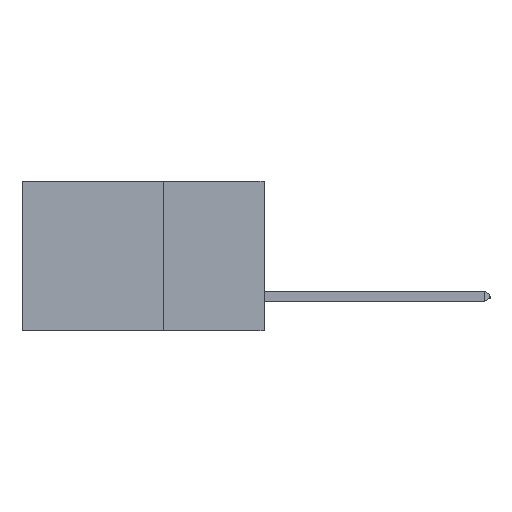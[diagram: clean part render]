
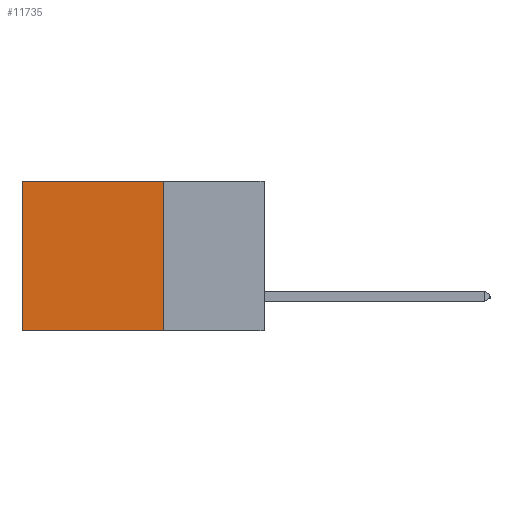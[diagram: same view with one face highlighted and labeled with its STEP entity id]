
A CAD part, left-side view. The second image highlights one B-rep face of the part: STEP entity #11735.
In plain terms, the highlighted planar face has unit normal (-1, 0, 0).
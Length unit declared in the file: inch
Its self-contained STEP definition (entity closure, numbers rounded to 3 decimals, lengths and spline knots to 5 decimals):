
#610 = DIRECTION ( 'NONE',  ( 1., 0., 0. ) ) ;
#1076 = ORIENTED_EDGE ( 'NONE', *, *, #19796, .F. ) ;
#1731 = EDGE_CURVE ( 'NONE', #18436, #6608, #20832, .T. ) ;
#1737 = DIRECTION ( 'NONE',  ( 0., 1., 0. ) ) ;
#3553 = VECTOR ( 'NONE', #10445, 39.37008 ) ;
#3681 = CARTESIAN_POINT ( 'NONE',  ( 0.298, 0.6, 0. ) ) ;
#4380 = VECTOR ( 'NONE', #1737, 39.37008 ) ;
#4457 = EDGE_CURVE ( 'NONE', #14496, #6608, #18977, .T. ) ;
#5786 = VERTEX_POINT ( 'NONE', #20628 ) ;
#6570 = CARTESIAN_POINT ( 'NONE',  ( 0.298, 0.25, 0. ) ) ;
#6608 = VERTEX_POINT ( 'NONE', #17324 ) ;
#7414 = CARTESIAN_POINT ( 'NONE',  ( 0.298, 0.6, 0. ) ) ;
#8276 = DIRECTION ( 'NONE',  ( 0., 0., -1. ) ) ;
#8797 = LINE ( 'NONE', #6570, #21544 ) ;
#8885 = LINE ( 'NONE', #12066, #4380 ) ;
#9000 = EDGE_LOOP ( 'NONE', ( #15523, #20691, #1076, #19505 ) ) ;
#9516 = CARTESIAN_POINT ( 'NONE',  ( 0.298, 0.25, -0.37 ) ) ;
#10445 = DIRECTION ( 'NONE',  ( 0., 1., 0. ) ) ;
#10496 = CARTESIAN_POINT ( 'NONE',  ( 0.298, 0.25, -0.37 ) ) ;
#11113 = CARTESIAN_POINT ( 'NONE',  ( 0.298, 0.25, 0. ) ) ;
#11735 = ADVANCED_FACE ( 'NONE', ( #21184 ), #19786, .F. ) ;
#12066 = CARTESIAN_POINT ( 'NONE',  ( 0.298, 0.25, 0. ) ) ;
#12870 = DIRECTION ( 'NONE',  ( 0., 0., -1. ) ) ;
#14496 = VERTEX_POINT ( 'NONE', #3681 ) ;
#15146 = EDGE_CURVE ( 'NONE', #5786, #14496, #8885, .T. ) ;
#15523 = ORIENTED_EDGE ( 'NONE', *, *, #4457, .T. ) ;
#17324 = CARTESIAN_POINT ( 'NONE',  ( 0.298, 0.6, -0.37 ) ) ;
#17369 = VECTOR ( 'NONE', #19507, 39.37008 ) ;
#18436 = VERTEX_POINT ( 'NONE', #9516 ) ;
#18977 = LINE ( 'NONE', #7414, #17369 ) ;
#19505 = ORIENTED_EDGE ( 'NONE', *, *, #15146, .T. ) ;
#19507 = DIRECTION ( 'NONE',  ( 0., 0., -1. ) ) ;
#19786 = PLANE ( 'NONE',  #19868 ) ;
#19796 = EDGE_CURVE ( 'NONE', #5786, #18436, #8797, .T. ) ;
#19868 = AXIS2_PLACEMENT_3D ( 'NONE', #11113, #610, #12870 ) ;
#20628 = CARTESIAN_POINT ( 'NONE',  ( 0.298, 0.25, 0. ) ) ;
#20691 = ORIENTED_EDGE ( 'NONE', *, *, #1731, .F. ) ;
#20832 = LINE ( 'NONE', #10496, #3553 ) ;
#21184 = FACE_OUTER_BOUND ( 'NONE', #9000, .T. ) ;
#21544 = VECTOR ( 'NONE', #8276, 39.37008 ) ;
